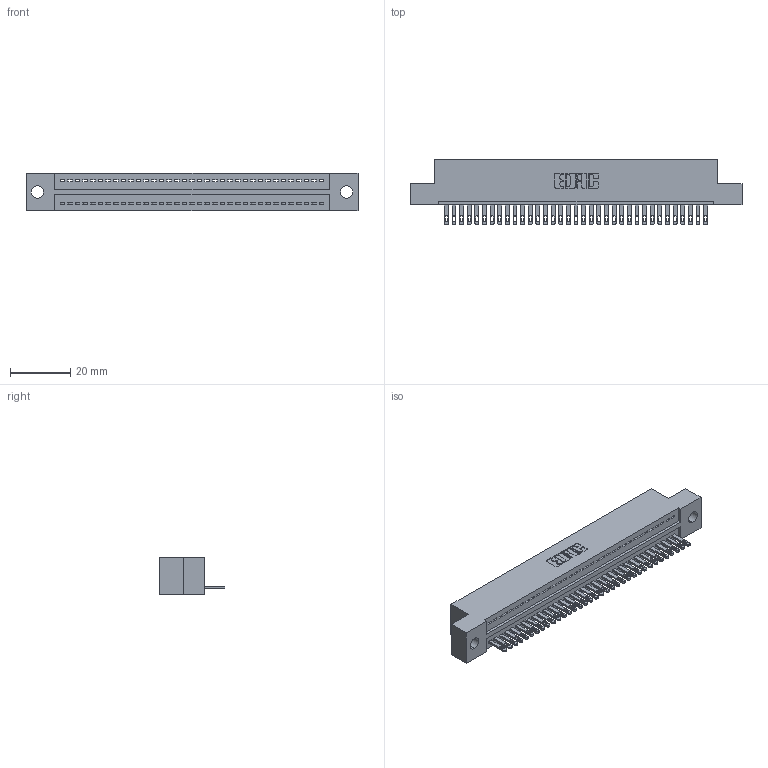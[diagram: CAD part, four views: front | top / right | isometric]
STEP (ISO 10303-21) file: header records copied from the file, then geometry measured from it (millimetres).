
FILE_DESCRIPTION (( 'STEP AP203' ), '1' );
FILE_NAME ('325-035-500-109.STEP', '2020-02-24T20:14:04', ( '' ), ( '' ), 'SwSTEP 2.0', 'SolidWorks 2016', '' );
FILE_SCHEMA (( 'CONFIG_CONTROL_DESIGN' ));
Length unit declared in the file: inch
Products named in the file (3): 325 Part_.160 TH; 325-035-500-109; 325-292-001_325-293-100
Assembly tree (36 placements, depth 2):
  325-035-500-109
    325 Part_.160 TH
    325-292-001_325-293-100  x35
Bounding box: 110.62 x 21.84 x 12.45 mm (x, y, z)
Volume: 13778.7 mm3; surface area: 14912.2 mm2
Topology: 36 solids, 36 shells, 2004 faces, 6191 edges, 4126 vertices
Faces by surface type: plane 1330, cylinder 674
Entity records: 22235 total; most frequent: CARTESIAN_POINT 3843, ORIENTED_EDGE 3814, DIRECTION 3257, EDGE_CURVE 1907, LINE 1775, VECTOR 1775, VERTEX_POINT 1270, AXIS2_PLACEMENT_3D 741
